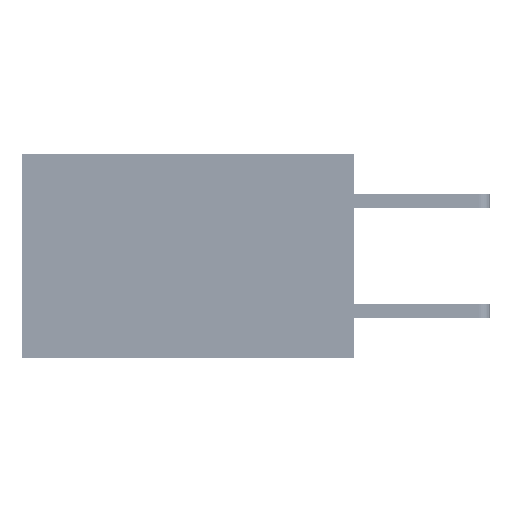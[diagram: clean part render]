
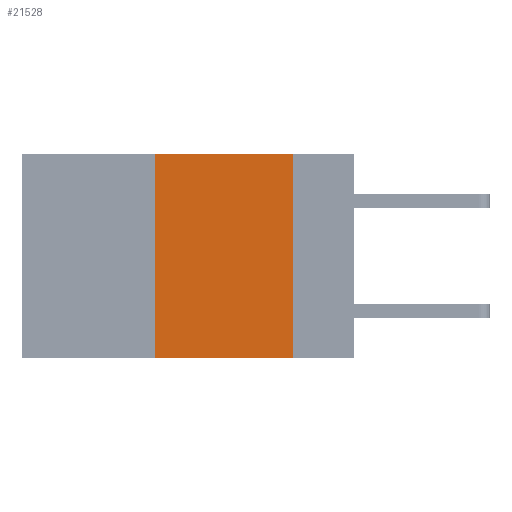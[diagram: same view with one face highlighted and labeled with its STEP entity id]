
A CAD part, left-side view. The second image highlights one B-rep face of the part: STEP entity #21528.
In plain terms, the highlighted planar face has unit normal (-1, 0, 0).
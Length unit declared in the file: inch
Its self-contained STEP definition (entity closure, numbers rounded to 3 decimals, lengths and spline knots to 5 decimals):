
#1259 = VERTEX_POINT ( 'NONE', #40569 ) ;
#2181 = VECTOR ( 'NONE', #30717, 39.37008 ) ;
#2664 = VECTOR ( 'NONE', #11892, 39.37008 ) ;
#4144 = VERTEX_POINT ( 'NONE', #11031 ) ;
#5071 = CARTESIAN_POINT ( 'NONE',  ( 0., 0.6, -0.37 ) ) ;
#5183 = DIRECTION ( 'NONE',  ( 1., 0., 0. ) ) ;
#9905 = VECTOR ( 'NONE', #25483, 39.37008 ) ;
#10460 = EDGE_CURVE ( 'NONE', #38353, #1259, #17004, .T. ) ;
#11031 = CARTESIAN_POINT ( 'NONE',  ( 0., 0.11, 0. ) ) ;
#11892 = DIRECTION ( 'NONE',  ( 0., 0., 1. ) ) ;
#14316 = AXIS2_PLACEMENT_3D ( 'NONE', #24153, #5183, #23860 ) ;
#15342 = VECTOR ( 'NONE', #24701, 39.37008 ) ;
#16324 = LINE ( 'NONE', #40572, #15342 ) ;
#17004 = LINE ( 'NONE', #40084, #2664 ) ;
#17887 = FACE_OUTER_BOUND ( 'NONE', #32736, .T. ) ;
#20560 = CARTESIAN_POINT ( 'NONE',  ( 0., 0.36, -0.37 ) ) ;
#21528 = ADVANCED_FACE ( 'NONE', ( #17887 ), #39601, .F. ) ;
#22252 = ORIENTED_EDGE ( 'NONE', *, *, #31598, .F. ) ;
#23860 = DIRECTION ( 'NONE',  ( 0., 0., -1. ) ) ;
#24153 = CARTESIAN_POINT ( 'NONE',  ( 0., 0.6, 0. ) ) ;
#24433 = VERTEX_POINT ( 'NONE', #40120 ) ;
#24701 = DIRECTION ( 'NONE',  ( 0., 0., -1. ) ) ;
#24947 = ORIENTED_EDGE ( 'NONE', *, *, #37398, .F. ) ;
#25483 = DIRECTION ( 'NONE',  ( 0., -1., 0. ) ) ;
#25611 = CARTESIAN_POINT ( 'NONE',  ( 0., 0.6, 0. ) ) ;
#26179 = EDGE_CURVE ( 'NONE', #38353, #24433, #30305, .T. ) ;
#27707 = LINE ( 'NONE', #25611, #9905 ) ;
#30305 = LINE ( 'NONE', #5071, #2181 ) ;
#30717 = DIRECTION ( 'NONE',  ( 0., -1., 0. ) ) ;
#31527 = ORIENTED_EDGE ( 'NONE', *, *, #26179, .T. ) ;
#31598 = EDGE_CURVE ( 'NONE', #4144, #24433, #16324, .T. ) ;
#32736 = EDGE_LOOP ( 'NONE', ( #22252, #24947, #34597, #31527 ) ) ;
#34597 = ORIENTED_EDGE ( 'NONE', *, *, #10460, .F. ) ;
#37398 = EDGE_CURVE ( 'NONE', #1259, #4144, #27707, .T. ) ;
#38353 = VERTEX_POINT ( 'NONE', #20560 ) ;
#39601 = PLANE ( 'NONE',  #14316 ) ;
#40084 = CARTESIAN_POINT ( 'NONE',  ( 0., 0.36, 0. ) ) ;
#40120 = CARTESIAN_POINT ( 'NONE',  ( 0., 0.11, -0.37 ) ) ;
#40569 = CARTESIAN_POINT ( 'NONE',  ( 0., 0.36, 0. ) ) ;
#40572 = CARTESIAN_POINT ( 'NONE',  ( 0., 0.11, 0. ) ) ;
